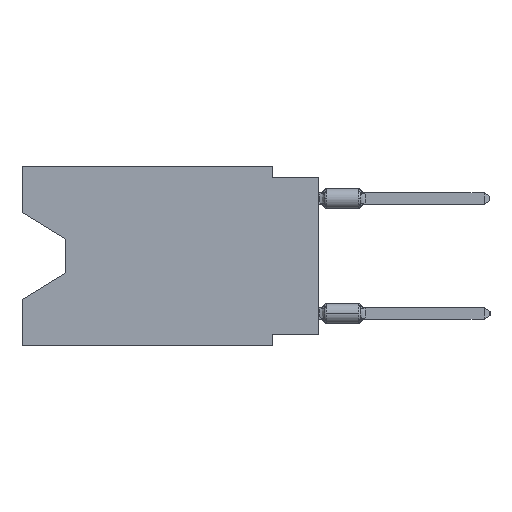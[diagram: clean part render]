
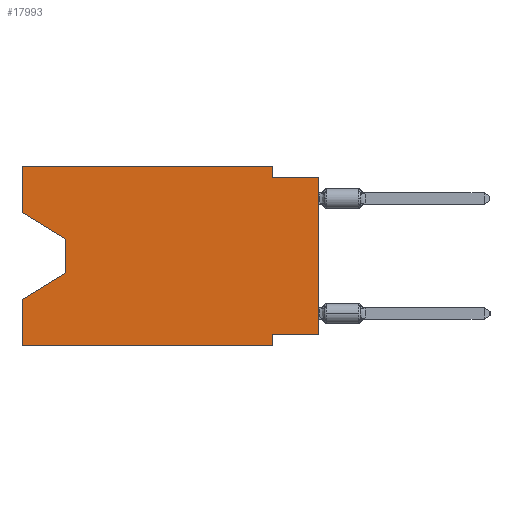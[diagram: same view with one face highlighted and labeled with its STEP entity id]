
A CAD part, left-side view. The second image highlights one B-rep face of the part: STEP entity #17993.
In plain terms, the highlighted planar face has unit normal (-1, 0, 0).
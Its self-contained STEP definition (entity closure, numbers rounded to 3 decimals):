
#256 = ORIENTED_EDGE ( 'NONE', *, *, #7429, .F. ) ;
#309 = ORIENTED_EDGE ( 'NONE', *, *, #10248, .T. ) ;
#415 = DIRECTION ( 'NONE',  ( 0., 0.855, -0.519 ) ) ;
#472 = DIRECTION ( 'NONE',  ( 0., 0., 1. ) ) ;
#558 = LINE ( 'NONE', #21957, #18649 ) ;
#1053 = DIRECTION ( 'NONE',  ( 0., 0., -1. ) ) ;
#1595 = VECTOR ( 'NONE', #21011, 1000. ) ;
#1882 = CARTESIAN_POINT ( 'NONE',  ( 0., 13.97, -4.013 ) ) ;
#2211 = ORIENTED_EDGE ( 'NONE', *, *, #17262, .T. ) ;
#2249 = EDGE_CURVE ( 'NONE', #22795, #28109, #24625, .T. ) ;
#2275 = FACE_OUTER_BOUND ( 'NONE', #10946, .T. ) ;
#2418 = EDGE_CURVE ( 'NONE', #6960, #19101, #28046, .T. ) ;
#2902 = VECTOR ( 'NONE', #472, 1000. ) ;
#3088 = CARTESIAN_POINT ( 'NONE',  ( 0., 16.383, -7.36 ) ) ;
#3174 = LINE ( 'NONE', #27022, #14886 ) ;
#3557 = VERTEX_POINT ( 'NONE', #12393 ) ;
#3792 = EDGE_CURVE ( 'NONE', #3557, #25183, #26467, .T. ) ;
#4351 = CARTESIAN_POINT ( 'NONE',  ( 0., 16.383, -9.906 ) ) ;
#4702 = LINE ( 'NONE', #6719, #14054 ) ;
#4869 = CARTESIAN_POINT ( 'NONE',  ( 0., 2.54, 0. ) ) ;
#5462 = DIRECTION ( 'NONE',  ( 0., 0., -1. ) ) ;
#5886 = DIRECTION ( 'NONE',  ( 0., -1., 0. ) ) ;
#6682 = DIRECTION ( 'NONE',  ( 0., 0., 1. ) ) ;
#6719 = CARTESIAN_POINT ( 'NONE',  ( 0., 0., -0.635 ) ) ;
#6859 = CARTESIAN_POINT ( 'NONE',  ( 0., 16.383, 0. ) ) ;
#6960 = VERTEX_POINT ( 'NONE', #4869 ) ;
#7229 = CARTESIAN_POINT ( 'NONE',  ( 0., 0., -9.271 ) ) ;
#7429 = EDGE_CURVE ( 'NONE', #28109, #14532, #18563, .T. ) ;
#8478 = DIRECTION ( 'NONE',  ( 0., 0., -1. ) ) ;
#8816 = CARTESIAN_POINT ( 'NONE',  ( 0., 0., 0. ) ) ;
#9188 = CARTESIAN_POINT ( 'NONE',  ( 0., 16.383, 0. ) ) ;
#9190 = EDGE_CURVE ( 'NONE', #25183, #6960, #16503, .T. ) ;
#10109 = AXIS2_PLACEMENT_3D ( 'NONE', #6859, #13041, #25990 ) ;
#10164 = CARTESIAN_POINT ( 'NONE',  ( 0., 0., -0.635 ) ) ;
#10189 = VERTEX_POINT ( 'NONE', #13342 ) ;
#10202 = VECTOR ( 'NONE', #15143, 1000. ) ;
#10248 = EDGE_CURVE ( 'NONE', #15355, #10189, #3174, .T. ) ;
#10843 = LINE ( 'NONE', #24211, #10202 ) ;
#10946 = EDGE_LOOP ( 'NONE', ( #18735, #309, #27014, #27990, #18866, #256, #18657, #2211, #14423, #13809, #17956, #11776 ) ) ;
#11043 = VECTOR ( 'NONE', #1053, 1000. ) ;
#11138 = VECTOR ( 'NONE', #6682, 1000. ) ;
#11776 = ORIENTED_EDGE ( 'NONE', *, *, #3792, .F. ) ;
#12005 = VECTOR ( 'NONE', #13683, 1000. ) ;
#12393 = CARTESIAN_POINT ( 'NONE',  ( 0., 16.383, -2.546 ) ) ;
#12893 = PLANE ( 'NONE',  #10109 ) ;
#13041 = DIRECTION ( 'NONE',  ( 1., 0., 0. ) ) ;
#13342 = CARTESIAN_POINT ( 'NONE',  ( 0., 13.97, -5.893 ) ) ;
#13579 = CARTESIAN_POINT ( 'NONE',  ( 0., 2.54, -9.271 ) ) ;
#13683 = DIRECTION ( 'NONE',  ( 0., 1., 0. ) ) ;
#13809 = ORIENTED_EDGE ( 'NONE', *, *, #2418, .F. ) ;
#14054 = VECTOR ( 'NONE', #15476, 1000. ) ;
#14423 = ORIENTED_EDGE ( 'NONE', *, *, #25613, .F. ) ;
#14532 = VERTEX_POINT ( 'NONE', #27560 ) ;
#14886 = VECTOR ( 'NONE', #5462, 1000. ) ;
#15044 = LINE ( 'NONE', #19223, #20519 ) ;
#15143 = DIRECTION ( 'NONE',  ( 0., 0., 1. ) ) ;
#15355 = VERTEX_POINT ( 'NONE', #1882 ) ;
#15476 = DIRECTION ( 'NONE',  ( 0., -1., 0. ) ) ;
#15862 = CARTESIAN_POINT ( 'NONE',  ( 0., 16.383, -2.546 ) ) ;
#15965 = VERTEX_POINT ( 'NONE', #4351 ) ;
#16503 = LINE ( 'NONE', #25283, #17035 ) ;
#16712 = VERTEX_POINT ( 'NONE', #10164 ) ;
#17035 = VECTOR ( 'NONE', #5886, 1000. ) ;
#17194 = EDGE_CURVE ( 'NONE', #15965, #19645, #10843, .T. ) ;
#17205 = DIRECTION ( 'NONE',  ( 0., -1., 0. ) ) ;
#17262 = EDGE_CURVE ( 'NONE', #22795, #16712, #25804, .T. ) ;
#17956 = ORIENTED_EDGE ( 'NONE', *, *, #9190, .F. ) ;
#17993 = ADVANCED_FACE ( 'NONE', ( #2275 ), #12893, .F. ) ;
#18563 = LINE ( 'NONE', #22882, #11043 ) ;
#18649 = VECTOR ( 'NONE', #415, 1000. ) ;
#18657 = ORIENTED_EDGE ( 'NONE', *, *, #2249, .F. ) ;
#18735 = ORIENTED_EDGE ( 'NONE', *, *, #21463, .T. ) ;
#18866 = ORIENTED_EDGE ( 'NONE', *, *, #24204, .T. ) ;
#19101 = VERTEX_POINT ( 'NONE', #26126 ) ;
#19223 = CARTESIAN_POINT ( 'NONE',  ( 0., 16.383, -9.906 ) ) ;
#19563 = CARTESIAN_POINT ( 'NONE',  ( 0., 2.54, 0. ) ) ;
#19645 = VERTEX_POINT ( 'NONE', #3088 ) ;
#20519 = VECTOR ( 'NONE', #17205, 1000. ) ;
#21011 = DIRECTION ( 'NONE',  ( 0., -0.855, -0.519 ) ) ;
#21463 = EDGE_CURVE ( 'NONE', #3557, #15355, #22480, .T. ) ;
#21957 = CARTESIAN_POINT ( 'NONE',  ( 0., 13.97, -5.893 ) ) ;
#22480 = LINE ( 'NONE', #15862, #1595 ) ;
#22795 = VERTEX_POINT ( 'NONE', #27221 ) ;
#22882 = CARTESIAN_POINT ( 'NONE',  ( 0., 2.54, -9.906 ) ) ;
#23917 = VECTOR ( 'NONE', #8478, 1000. ) ;
#24204 = EDGE_CURVE ( 'NONE', #15965, #14532, #15044, .T. ) ;
#24211 = CARTESIAN_POINT ( 'NONE',  ( 0., 16.383, 0. ) ) ;
#24625 = LINE ( 'NONE', #7229, #12005 ) ;
#25183 = VERTEX_POINT ( 'NONE', #26297 ) ;
#25283 = CARTESIAN_POINT ( 'NONE',  ( 0., 16.383, 0. ) ) ;
#25480 = EDGE_CURVE ( 'NONE', #10189, #19645, #558, .T. ) ;
#25613 = EDGE_CURVE ( 'NONE', #19101, #16712, #4702, .T. ) ;
#25804 = LINE ( 'NONE', #8816, #11138 ) ;
#25990 = DIRECTION ( 'NONE',  ( 0., 0., -1. ) ) ;
#26126 = CARTESIAN_POINT ( 'NONE',  ( 0., 2.54, -0.635 ) ) ;
#26297 = CARTESIAN_POINT ( 'NONE',  ( 0., 16.383, 0. ) ) ;
#26467 = LINE ( 'NONE', #9188, #2902 ) ;
#27014 = ORIENTED_EDGE ( 'NONE', *, *, #25480, .T. ) ;
#27022 = CARTESIAN_POINT ( 'NONE',  ( 0., 13.97, -4.013 ) ) ;
#27221 = CARTESIAN_POINT ( 'NONE',  ( 0., 0., -9.271 ) ) ;
#27560 = CARTESIAN_POINT ( 'NONE',  ( 0., 2.54, -9.906 ) ) ;
#27990 = ORIENTED_EDGE ( 'NONE', *, *, #17194, .F. ) ;
#28046 = LINE ( 'NONE', #19563, #23917 ) ;
#28109 = VERTEX_POINT ( 'NONE', #13579 ) ;
